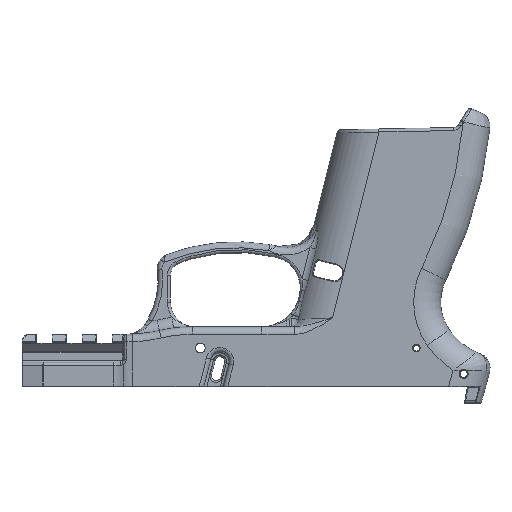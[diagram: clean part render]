
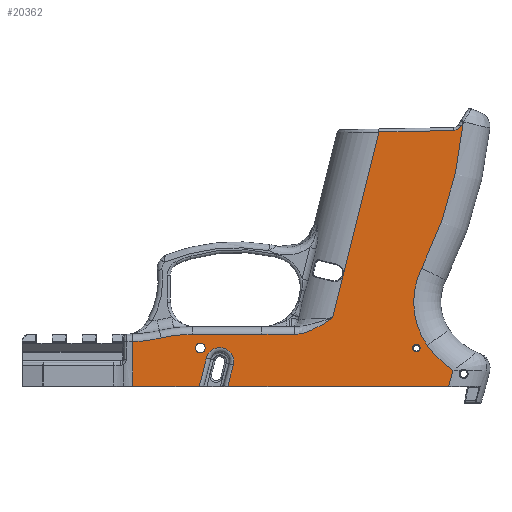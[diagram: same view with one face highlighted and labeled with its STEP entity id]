
A CAD part, front view. The second image highlights one B-rep face of the part: STEP entity #20362.
In plain terms, the highlighted planar face has unit normal (0, -1, 0).
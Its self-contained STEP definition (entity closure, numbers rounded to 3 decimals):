
#364=FACE_BOUND('',#3328,.T.);
#365=FACE_BOUND('',#3329,.T.);
#382=PLANE('',#21675);
#587=B_SPLINE_CURVE_WITH_KNOTS('',3,(#30437,#30438,#30439,#30440,#30441,
#30442,#30443,#30444,#30445,#30446),.UNSPECIFIED.,.F.,.F.,(4,1,1,1,1,2,
4),(0.,0.279,0.559,0.838,1.117,
1.396,1.398),.UNSPECIFIED.);
#2062=FACE_OUTER_BOUND('',#3327,.T.);
#3327=EDGE_LOOP('',(#13254,#13255,#13256,#13257,#13258,#13259,#13260,#13261,
#13262,#13263,#13264,#13265,#13266,#13267,#13268,#13269,#13270,#13271,#13272));
#3328=EDGE_LOOP('',(#13273));
#3329=EDGE_LOOP('',(#13274));
#4627=LINE('',#30379,#5678);
#4629=LINE('',#30401,#5680);
#4631=LINE('',#30413,#5682);
#4632=LINE('',#30417,#5683);
#4633=LINE('',#30419,#5684);
#4634=LINE('',#30421,#5685);
#4635=LINE('',#30429,#5686);
#4636=LINE('',#30433,#5687);
#4637=LINE('',#30435,#5688);
#4638=LINE('',#30448,#5689);
#4639=LINE('',#30450,#5690);
#5678=VECTOR('',#24179,1000.);
#5680=VECTOR('',#24187,10.);
#5682=VECTOR('',#24201,1000.);
#5683=VECTOR('',#24204,1000.);
#5684=VECTOR('',#24205,1000.);
#5685=VECTOR('',#24206,1000.);
#5686=VECTOR('',#24213,1000.);
#5687=VECTOR('',#24216,1000.);
#5688=VECTOR('',#24217,1000.);
#5689=VECTOR('',#24218,1000.);
#5690=VECTOR('',#24219,1000.);
#6721=CIRCLE('',#21672,1.6);
#6724=CIRCLE('',#21676,50.431);
#6725=CIRCLE('',#21677,4.625);
#6726=CIRCLE('',#21678,30.273);
#6727=CIRCLE('',#21679,25.273);
#6728=CIRCLE('',#21680,136.);
#6729=CIRCLE('',#21681,3.);
#6730=CIRCLE('',#21682,45.431);
#6731=CIRCLE('',#21683,1.25);
#7811=VERTEX_POINT('',#30353);
#7817=VERTEX_POINT('',#30377);
#7819=VERTEX_POINT('',#30382);
#7822=VERTEX_POINT('',#30399);
#7823=VERTEX_POINT('',#30403);
#7826=VERTEX_POINT('',#30411);
#7827=VERTEX_POINT('',#30414);
#7828=VERTEX_POINT('',#30416);
#7829=VERTEX_POINT('',#30418);
#7830=VERTEX_POINT('',#30420);
#7831=VERTEX_POINT('',#30422);
#7832=VERTEX_POINT('',#30424);
#7833=VERTEX_POINT('',#30426);
#7834=VERTEX_POINT('',#30428);
#7835=VERTEX_POINT('',#30430);
#7836=VERTEX_POINT('',#30432);
#7837=VERTEX_POINT('',#30434);
#7838=VERTEX_POINT('',#30436);
#7839=VERTEX_POINT('',#30447);
#7840=VERTEX_POINT('',#30449);
#7841=VERTEX_POINT('',#30452);
#9894=EDGE_CURVE('',#7817,#7811,#4627,.T.);
#9899=EDGE_CURVE('',#7819,#7822,#4629,.T.);
#9900=EDGE_CURVE('',#7823,#7823,#6721,.T.);
#9904=EDGE_CURVE('',#7811,#7826,#6724,.T.);
#9905=EDGE_CURVE('',#7819,#7817,#4631,.T.);
#9906=EDGE_CURVE('',#7827,#7822,#6725,.T.);
#9907=EDGE_CURVE('',#7828,#7827,#4632,.T.);
#9908=EDGE_CURVE('',#7829,#7828,#4633,.T.);
#9909=EDGE_CURVE('',#7830,#7829,#4634,.T.);
#9910=EDGE_CURVE('',#7831,#7830,#6726,.T.);
#9911=EDGE_CURVE('',#7832,#7831,#6727,.T.);
#9912=EDGE_CURVE('',#7832,#7833,#6728,.T.);
#9913=EDGE_CURVE('',#7833,#7834,#4635,.T.);
#9914=EDGE_CURVE('',#7835,#7834,#6729,.T.);
#9915=EDGE_CURVE('',#7835,#7836,#4636,.T.);
#9916=EDGE_CURVE('',#7836,#7837,#4637,.T.);
#9917=EDGE_CURVE('',#7838,#7837,#587,.T.);
#9918=EDGE_CURVE('',#7839,#7838,#4638,.T.);
#9919=EDGE_CURVE('',#7840,#7839,#4639,.T.);
#9920=EDGE_CURVE('',#7840,#7826,#6730,.T.);
#9921=EDGE_CURVE('',#7841,#7841,#6731,.T.);
#13254=ORIENTED_EDGE('',*,*,#9904,.F.);
#13255=ORIENTED_EDGE('',*,*,#9894,.F.);
#13256=ORIENTED_EDGE('',*,*,#9905,.F.);
#13257=ORIENTED_EDGE('',*,*,#9899,.T.);
#13258=ORIENTED_EDGE('',*,*,#9906,.F.);
#13259=ORIENTED_EDGE('',*,*,#9907,.F.);
#13260=ORIENTED_EDGE('',*,*,#9908,.F.);
#13261=ORIENTED_EDGE('',*,*,#9909,.F.);
#13262=ORIENTED_EDGE('',*,*,#9910,.F.);
#13263=ORIENTED_EDGE('',*,*,#9911,.F.);
#13264=ORIENTED_EDGE('',*,*,#9912,.T.);
#13265=ORIENTED_EDGE('',*,*,#9913,.T.);
#13266=ORIENTED_EDGE('',*,*,#9914,.F.);
#13267=ORIENTED_EDGE('',*,*,#9915,.T.);
#13268=ORIENTED_EDGE('',*,*,#9916,.T.);
#13269=ORIENTED_EDGE('',*,*,#9917,.F.);
#13270=ORIENTED_EDGE('',*,*,#9918,.F.);
#13271=ORIENTED_EDGE('',*,*,#9919,.F.);
#13272=ORIENTED_EDGE('',*,*,#9920,.T.);
#13273=ORIENTED_EDGE('',*,*,#9900,.T.);
#13274=ORIENTED_EDGE('',*,*,#9921,.F.);
#20362=ADVANCED_FACE('',(#2062,#364,#365),#382,.F.);
#21672=AXIS2_PLACEMENT_3D('',#30404,#24190,#24191);
#21675=AXIS2_PLACEMENT_3D('',#30410,#24197,#24198);
#21676=AXIS2_PLACEMENT_3D('',#30412,#24199,#24200);
#21677=AXIS2_PLACEMENT_3D('',#30415,#24202,#24203);
#21678=AXIS2_PLACEMENT_3D('',#30423,#24207,#24208);
#21679=AXIS2_PLACEMENT_3D('',#30425,#24209,#24210);
#21680=AXIS2_PLACEMENT_3D('',#30427,#24211,#24212);
#21681=AXIS2_PLACEMENT_3D('',#30431,#24214,#24215);
#21682=AXIS2_PLACEMENT_3D('',#30451,#24220,#24221);
#21683=AXIS2_PLACEMENT_3D('',#30453,#24222,#24223);
#24179=DIRECTION('',(0.,0.,1.));
#24187=DIRECTION('',(0.25,0.,0.968));
#24190=DIRECTION('center_axis',(0.,1.,0.));
#24191=DIRECTION('ref_axis',(1.,0.,0.));
#24197=DIRECTION('center_axis',(0.,1.,0.));
#24198=DIRECTION('ref_axis',(1.,0.,0.));
#24199=DIRECTION('center_axis',(0.,-1.,0.));
#24200=DIRECTION('ref_axis',(0.,0.,1.));
#24201=DIRECTION('',(-1.,0.,0.));
#24202=DIRECTION('center_axis',(0.,-1.,0.));
#24203=DIRECTION('ref_axis',(0.25,0.,0.968));
#24204=DIRECTION('',(0.25,0.,0.968));
#24205=DIRECTION('',(-1.,0.,0.));
#24206=DIRECTION('',(-0.259,0.,-0.966));
#24207=DIRECTION('center_axis',(0.,-1.,0.));
#24208=DIRECTION('ref_axis',(-0.614,0.,-0.79));
#24209=DIRECTION('center_axis',(0.,-1.,0.));
#24210=DIRECTION('ref_axis',(-0.894,0.,0.448));
#24211=DIRECTION('center_axis',(0.,-1.,0.));
#24212=DIRECTION('ref_axis',(0.894,0.,-0.448));
#24213=DIRECTION('',(-0.537,0.,-0.843));
#24214=DIRECTION('center_axis',(0.,-1.,0.));
#24215=DIRECTION('ref_axis',(0.02,0.,-1.));
#24216=DIRECTION('',(-1.,0.,-0.02));
#24217=DIRECTION('',(-0.242,0.,-0.97));
#24218=DIRECTION('',(1.,0.,0.));
#24219=DIRECTION('',(1.,0.,0.));
#24220=DIRECTION('center_axis',(0.,-1.,0.));
#24221=DIRECTION('ref_axis',(0.,0.,-1.));
#24222=DIRECTION('center_axis',(0.,-1.,0.));
#24223=DIRECTION('ref_axis',(1.,0.,0.));
#30353=CARTESIAN_POINT('',(-41.114,-13.5,-22.465));
#30377=CARTESIAN_POINT('',(-41.114,-13.5,-37.26));
#30379=CARTESIAN_POINT('',(-41.114,-13.5,0.));
#30382=CARTESIAN_POINT('',(-18.901,-13.5,-37.26));
#30399=CARTESIAN_POINT('',(-16.478,-13.5,-27.878));
#30401=CARTESIAN_POINT('',(-12.139,-13.5,-11.074));
#30403=CARTESIAN_POINT('',(-20.125,-13.5,-24.534));
#30404=CARTESIAN_POINT('Origin',(-18.525,-13.5,-24.534));
#30410=CARTESIAN_POINT('Origin',(0.169,-13.5,8.836));
#30411=CARTESIAN_POINT('',(-31.558,-13.5,-21.185));
#30412=CARTESIAN_POINT('Origin',(-43.,-13.5,27.931));
#30413=CARTESIAN_POINT('',(38.335,-13.5,-37.26));
#30414=CARTESIAN_POINT('',(-7.522,-13.5,-30.19));
#30415=CARTESIAN_POINT('Origin',(-12.,-13.5,-29.034));
#30416=CARTESIAN_POINT('',(-9.347,-13.5,-37.26));
#30417=CARTESIAN_POINT('',(-2.558,-13.5,-10.966));
#30418=CARTESIAN_POINT('',(64.275,-13.5,-37.26));
#30419=CARTESIAN_POINT('',(38.335,-13.5,-37.26));
#30420=CARTESIAN_POINT('',(65.709,-13.5,-31.909));
#30421=CARTESIAN_POINT('',(68.907,-13.5,-19.972));
#30422=CARTESIAN_POINT('',(57.113,-13.5,-23.628));
#30423=CARTESIAN_POINT('Origin',(82.001,-13.5,-6.394));
#30424=CARTESIAN_POINT('',(55.298,-13.5,2.087));
#30425=CARTESIAN_POINT('Origin',(77.891,-13.5,-9.24));
#30426=CARTESIAN_POINT('',(69.152,-13.5,50.609));
#30427=CARTESIAN_POINT('Origin',(-66.279,-13.5,63.039));
#30428=CARTESIAN_POINT('',(68.36,-13.5,49.366));
#30429=CARTESIAN_POINT('',(69.152,-13.5,50.609));
#30430=CARTESIAN_POINT('',(65.89,-13.5,47.979));
#30431=CARTESIAN_POINT('Origin',(65.83,-13.5,50.978));
#30432=CARTESIAN_POINT('',(41.001,-13.5,47.481));
#30433=CARTESIAN_POINT('',(65.89,-13.5,47.979));
#30434=CARTESIAN_POINT('',(25.548,-13.5,-14.5));
#30435=CARTESIAN_POINT('',(41.001,-13.5,47.481));
#30436=CARTESIAN_POINT('',(12.873,-13.5,-20.));
#30437=CARTESIAN_POINT('Ctrl Pts',(12.873,-13.5,-20.));
#30438=CARTESIAN_POINT('Ctrl Pts',(13.804,-13.5,-20.));
#30439=CARTESIAN_POINT('Ctrl Pts',(15.679,-13.5,-19.742));
#30440=CARTESIAN_POINT('Ctrl Pts',(18.327,-13.5,-18.821));
#30441=CARTESIAN_POINT('Ctrl Pts',(20.817,-13.5,-17.56));
#30442=CARTESIAN_POINT('Ctrl Pts',(23.213,-13.5,-16.079));
#30443=CARTESIAN_POINT('Ctrl Pts',(24.765,-13.5,-15.029));
#30444=CARTESIAN_POINT('Ctrl Pts',(25.54,-13.5,-14.505));
#30445=CARTESIAN_POINT('Ctrl Pts',(25.544,-13.5,-14.502));
#30446=CARTESIAN_POINT('Ctrl Pts',(25.548,-13.5,-14.5));
#30447=CARTESIAN_POINT('',(2.,-13.5,-20.));
#30448=CARTESIAN_POINT('',(1.085,-13.5,-20.));
#30449=CARTESIAN_POINT('',(-21.25,-13.5,-20.));
#30450=CARTESIAN_POINT('',(1.085,-13.5,-20.));
#30451=CARTESIAN_POINT('Origin',(-21.25,-13.5,-65.431));
#30452=CARTESIAN_POINT('',(52.3,-13.5,-24.575));
#30453=CARTESIAN_POINT('Origin',(53.55,-13.5,-24.575));
